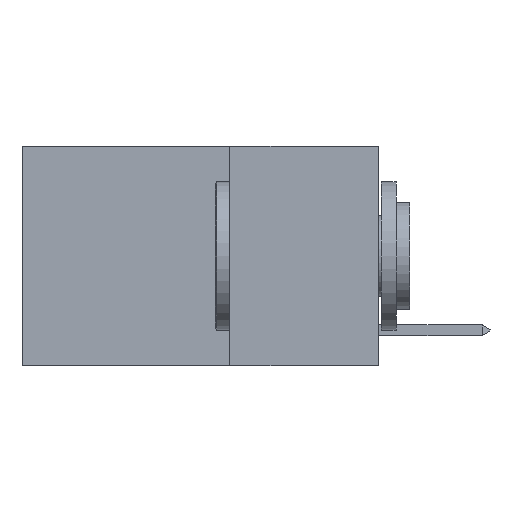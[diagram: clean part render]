
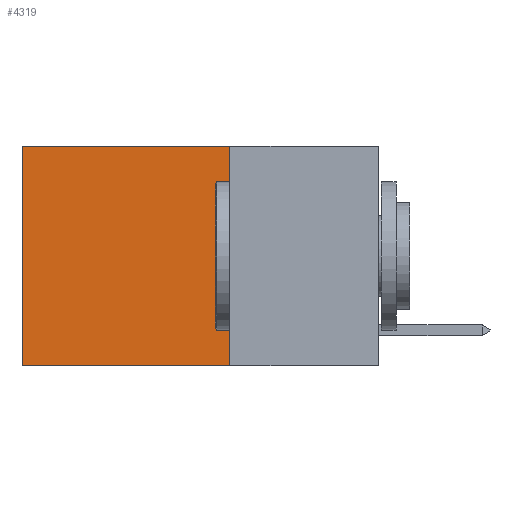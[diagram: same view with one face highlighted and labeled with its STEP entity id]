
A CAD part, left-side view. The second image highlights one B-rep face of the part: STEP entity #4319.
In plain terms, the highlighted planar face has unit normal (-1, 0, 0).
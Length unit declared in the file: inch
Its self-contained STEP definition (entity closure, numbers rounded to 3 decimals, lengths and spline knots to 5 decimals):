
#2169 = AXIS2_PLACEMENT_3D ( 'NONE', #24358, #5229, #5408 ) ;
#3532 = EDGE_LOOP ( 'NONE', ( #18774, #23500, #10762, #7941 ) ) ;
#3550 = CARTESIAN_POINT ( 'NONE',  ( 0.2625, 0.6, 0. ) ) ;
#3555 = CARTESIAN_POINT ( 'NONE',  ( 0.2625, 0.25, 0. ) ) ;
#4001 = VERTEX_POINT ( 'NONE', #6739 ) ;
#4040 = DIRECTION ( 'NONE',  ( 0., 1., 0. ) ) ;
#4319 = ADVANCED_FACE ( 'NONE', ( #6779 ), #22236, .F. ) ;
#4464 = CARTESIAN_POINT ( 'NONE',  ( 0.2625, 0.6, -0.37 ) ) ;
#5229 = DIRECTION ( 'NONE',  ( 1., 0., 0. ) ) ;
#5408 = DIRECTION ( 'NONE',  ( 0., 0., -1. ) ) ;
#6306 = CARTESIAN_POINT ( 'NONE',  ( 0.2625, 0.25, 0. ) ) ;
#6739 = CARTESIAN_POINT ( 'NONE',  ( 0.2625, 0.25, -0.37 ) ) ;
#6779 = FACE_OUTER_BOUND ( 'NONE', #3532, .T. ) ;
#7217 = CARTESIAN_POINT ( 'NONE',  ( 0.2625, 0.25, 0. ) ) ;
#7941 = ORIENTED_EDGE ( 'NONE', *, *, #16558, .T. ) ;
#9408 = LINE ( 'NONE', #6306, #12812 ) ;
#9849 = DIRECTION ( 'NONE',  ( 0., 0., -1. ) ) ;
#10710 = CARTESIAN_POINT ( 'NONE',  ( 0.2625, 0.6, 0. ) ) ;
#10762 = ORIENTED_EDGE ( 'NONE', *, *, #20856, .F. ) ;
#11432 = VECTOR ( 'NONE', #9849, 39.37008 ) ;
#12588 = VERTEX_POINT ( 'NONE', #4464 ) ;
#12598 = VECTOR ( 'NONE', #14460, 39.37008 ) ;
#12812 = VECTOR ( 'NONE', #4040, 39.37008 ) ;
#12871 = VERTEX_POINT ( 'NONE', #10710 ) ;
#13811 = LINE ( 'NONE', #3555, #18116 ) ;
#14460 = DIRECTION ( 'NONE',  ( 0., 1., 0. ) ) ;
#14633 = VERTEX_POINT ( 'NONE', #7217 ) ;
#16558 = EDGE_CURVE ( 'NONE', #14633, #12871, #9408, .T. ) ;
#16581 = DIRECTION ( 'NONE',  ( 0., 0., -1. ) ) ;
#17882 = LINE ( 'NONE', #27317, #12598 ) ;
#18116 = VECTOR ( 'NONE', #16581, 39.37008 ) ;
#18774 = ORIENTED_EDGE ( 'NONE', *, *, #21442, .T. ) ;
#20856 = EDGE_CURVE ( 'NONE', #14633, #4001, #13811, .T. ) ;
#21442 = EDGE_CURVE ( 'NONE', #12871, #12588, #23121, .T. ) ;
#22236 = PLANE ( 'NONE',  #2169 ) ;
#23121 = LINE ( 'NONE', #3550, #11432 ) ;
#23500 = ORIENTED_EDGE ( 'NONE', *, *, #24477, .F. ) ;
#24358 = CARTESIAN_POINT ( 'NONE',  ( 0.2625, 0.25, 0. ) ) ;
#24477 = EDGE_CURVE ( 'NONE', #4001, #12588, #17882, .T. ) ;
#27317 = CARTESIAN_POINT ( 'NONE',  ( 0.2625, 0.25, -0.37 ) ) ;
